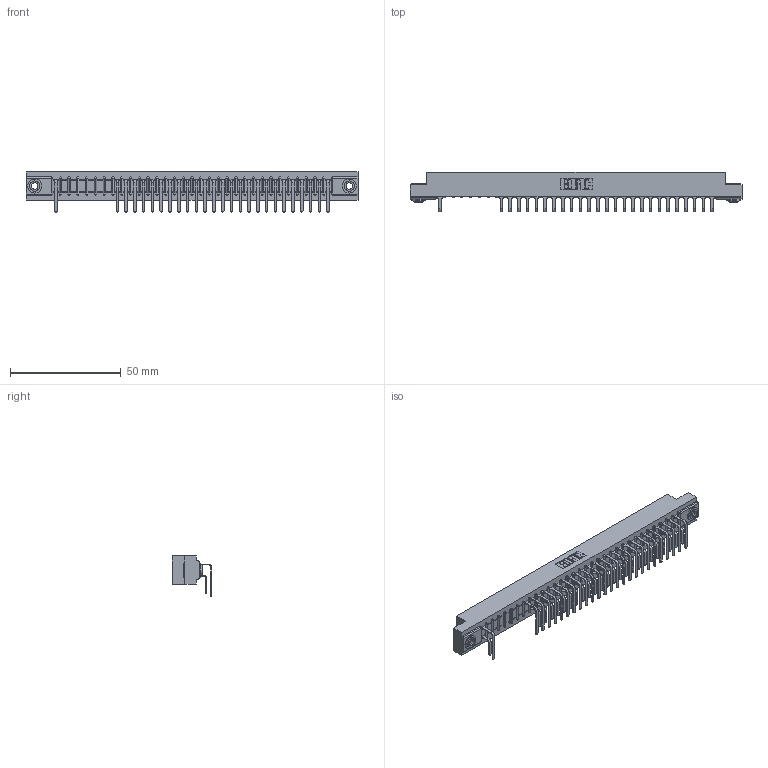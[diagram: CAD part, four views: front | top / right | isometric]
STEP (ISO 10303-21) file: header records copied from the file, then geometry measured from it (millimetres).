
FILE_DESCRIPTION (( 'STEP AP203' ), '1' );
FILE_NAME ('307-032-559-103.STEP', '2018-08-04T21:42:33', ( '' ), ( '' ), 'SwSTEP 2.0', 'SolidWorks 2016', '' );
FILE_SCHEMA (( 'CONFIG_CONTROL_DESIGN' ));
Length unit declared in the file: inch
Products named in the file (5): 345-250-002_345-250-002-102; 307-032-559-103; 307 Part_.156 Dia Mounting Holes; 307-290-001_558 559 - 1 (Single); 307-290-001_559 - 2 (Single)
Assembly tree (54 placements, depth 2):
  307-032-559-103
    307 Part_.156 Dia Mounting Holes
    307-290-001_558 559 - 1 (Single)  x25
    307-290-001_559 - 2 (Single)  x26
    345-250-002_345-250-002-102  x2
Bounding box: 149.81 x 17.69 x 18.07 mm (x, y, z)
Volume: 15920.3 mm3; surface area: 19750.8 mm2
Topology: 54 solids, 54 shells, 2883 faces, 8093 edges, 5234 vertices
Faces by surface type: plane 1855, cylinder 954, sphere 66, cone 8
Entity records: 31786 total; most frequent: CARTESIAN_POINT 5242, ORIENTED_EDGE 5198, DIRECTION 5139, EDGE_CURVE 2599, VECTOR 1981, LINE 1981, VERTEX_POINT 1682, AXIS2_PLACEMENT_3D 1579
